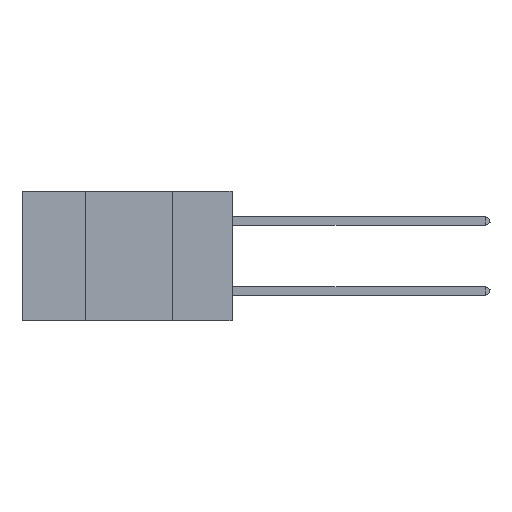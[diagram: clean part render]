
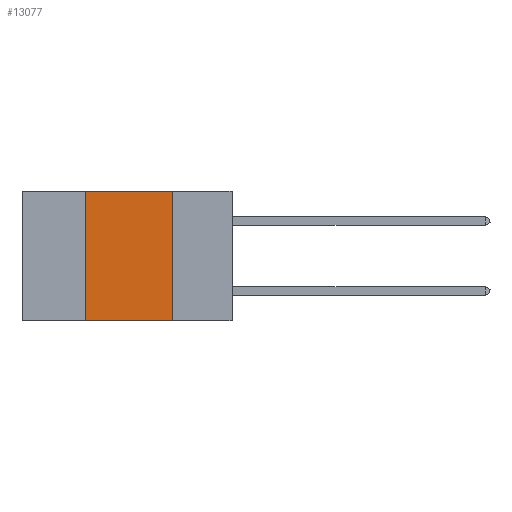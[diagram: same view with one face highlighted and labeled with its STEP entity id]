
A CAD part, left-side view. The second image highlights one B-rep face of the part: STEP entity #13077.
In plain terms, the highlighted planar face has unit normal (-1, 0, 0).
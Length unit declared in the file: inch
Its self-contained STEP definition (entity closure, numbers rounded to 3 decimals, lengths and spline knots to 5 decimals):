
#815 = EDGE_LOOP ( 'NONE', ( #14361, #11222, #20654, #6040 ) ) ;
#1689 = VECTOR ( 'NONE', #8774, 39.37008 ) ;
#2003 = DIRECTION ( 'NONE',  ( 0., 0., -1. ) ) ;
#2019 = LINE ( 'NONE', #15392, #19329 ) ;
#2087 = CARTESIAN_POINT ( 'NONE',  ( 0., 0.42, -0.37 ) ) ;
#2260 = LINE ( 'NONE', #20583, #1689 ) ;
#2383 = FACE_OUTER_BOUND ( 'NONE', #815, .T. ) ;
#3572 = CARTESIAN_POINT ( 'NONE',  ( 0., 0.17, 0. ) ) ;
#3695 = CARTESIAN_POINT ( 'NONE',  ( 0., 0.6, 0. ) ) ;
#4244 = VECTOR ( 'NONE', #2003, 39.37008 ) ;
#4297 = EDGE_CURVE ( 'NONE', #10403, #10253, #2019, .T. ) ;
#6040 = ORIENTED_EDGE ( 'NONE', *, *, #4297, .T. ) ;
#6720 = VERTEX_POINT ( 'NONE', #3572 ) ;
#7036 = AXIS2_PLACEMENT_3D ( 'NONE', #3695, #17467, #7307 ) ;
#7307 = DIRECTION ( 'NONE',  ( 0., 0., -1. ) ) ;
#7564 = EDGE_CURVE ( 'NONE', #8953, #6720, #21980, .T. ) ;
#8437 = LINE ( 'NONE', #14287, #4244 ) ;
#8538 = VECTOR ( 'NONE', #11187, 39.37008 ) ;
#8774 = DIRECTION ( 'NONE',  ( 0., 0., 1. ) ) ;
#8953 = VERTEX_POINT ( 'NONE', #21086 ) ;
#9011 = PLANE ( 'NONE',  #7036 ) ;
#10237 = EDGE_CURVE ( 'NONE', #10403, #8953, #2260, .T. ) ;
#10253 = VERTEX_POINT ( 'NONE', #15660 ) ;
#10381 = EDGE_CURVE ( 'NONE', #6720, #10253, #8437, .T. ) ;
#10403 = VERTEX_POINT ( 'NONE', #2087 ) ;
#11187 = DIRECTION ( 'NONE',  ( 0., -1., 0. ) ) ;
#11222 = ORIENTED_EDGE ( 'NONE', *, *, #7564, .F. ) ;
#12037 = DIRECTION ( 'NONE',  ( 0., -1., 0. ) ) ;
#12805 = CARTESIAN_POINT ( 'NONE',  ( 0., 0.6, 0. ) ) ;
#13077 = ADVANCED_FACE ( 'NONE', ( #2383 ), #9011, .F. ) ;
#14287 = CARTESIAN_POINT ( 'NONE',  ( 0., 0.17, 0. ) ) ;
#14361 = ORIENTED_EDGE ( 'NONE', *, *, #10381, .F. ) ;
#15392 = CARTESIAN_POINT ( 'NONE',  ( 0., 0.6, -0.37 ) ) ;
#15660 = CARTESIAN_POINT ( 'NONE',  ( 0., 0.17, -0.37 ) ) ;
#17467 = DIRECTION ( 'NONE',  ( 1., 0., 0. ) ) ;
#19329 = VECTOR ( 'NONE', #12037, 39.37008 ) ;
#20583 = CARTESIAN_POINT ( 'NONE',  ( 0., 0.42, 0. ) ) ;
#20654 = ORIENTED_EDGE ( 'NONE', *, *, #10237, .F. ) ;
#21086 = CARTESIAN_POINT ( 'NONE',  ( 0., 0.42, 0. ) ) ;
#21980 = LINE ( 'NONE', #12805, #8538 ) ;
